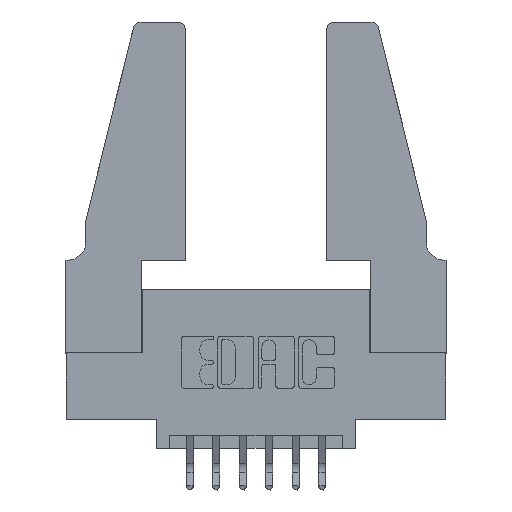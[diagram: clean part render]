
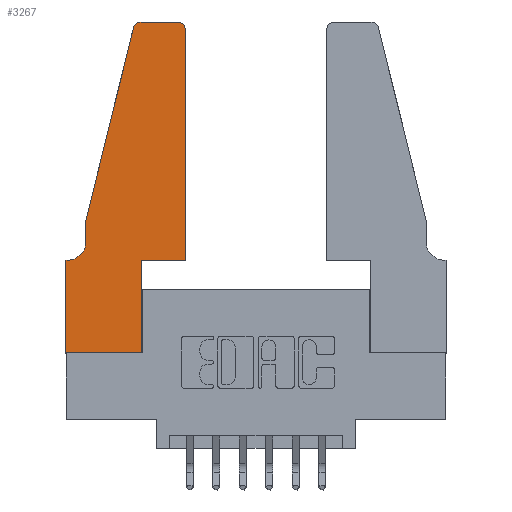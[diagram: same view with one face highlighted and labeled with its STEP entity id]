
A CAD part, top view. The second image highlights one B-rep face of the part: STEP entity #3267.
In plain terms, the highlighted planar face has unit normal (0, 0, 1).
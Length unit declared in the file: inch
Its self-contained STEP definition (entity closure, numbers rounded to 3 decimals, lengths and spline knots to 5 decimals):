
#171 = VECTOR ( 'NONE', #5055, 39.37008 ) ;
#303 = CARTESIAN_POINT ( 'NONE',  ( 0.4505, 1.22, 0.37 ) ) ;
#331 = CARTESIAN_POINT ( 'NONE',  ( 0.4505, 0.35, 0.37 ) ) ;
#343 = VERTEX_POINT ( 'NONE', #2088 ) ;
#432 = CARTESIAN_POINT ( 'NONE',  ( 0.284, 1.25, 0.37 ) ) ;
#476 = DIRECTION ( 'NONE',  ( 1., 0., 0. ) ) ;
#612 = CARTESIAN_POINT ( 'NONE',  ( 0.0055, 0.35, 0.37 ) ) ;
#624 = EDGE_CURVE ( 'NONE', #7523, #343, #2454, .T. ) ;
#1368 = EDGE_CURVE ( 'NONE', #3837, #6084, #7734, .T. ) ;
#1468 = DIRECTION ( 'NONE',  ( 0., 0., 1. ) ) ;
#1551 = VECTOR ( 'NONE', #6899, 39.37008 ) ;
#1742 = CIRCLE ( 'NONE', #3363, 0.03 ) ;
#1766 = LINE ( 'NONE', #4999, #3747 ) ;
#1780 = VERTEX_POINT ( 'NONE', #7003 ) ;
#1866 = ORIENTED_EDGE ( 'NONE', *, *, #7476, .T. ) ;
#2088 = CARTESIAN_POINT ( 'NONE',  ( 0.2865, 0.35, 0.37 ) ) ;
#2177 = DIRECTION ( 'NONE',  ( 0., 0., -1. ) ) ;
#2454 = LINE ( 'NONE', #7341, #4933 ) ;
#2511 = VECTOR ( 'NONE', #7193, 39.37008 ) ;
#2531 = ORIENTED_EDGE ( 'NONE', *, *, #624, .T. ) ;
#2634 = CARTESIAN_POINT ( 'NONE',  ( 0., 0., 0.37 ) ) ;
#2640 = LINE ( 'NONE', #2634, #2511 ) ;
#2693 = ORIENTED_EDGE ( 'NONE', *, *, #7391, .T. ) ;
#2748 = VERTEX_POINT ( 'NONE', #303 ) ;
#2749 = VERTEX_POINT ( 'NONE', #432 ) ;
#3013 = CARTESIAN_POINT ( 'NONE',  ( 0.25487, 1.22718, 0.37 ) ) ;
#3137 = DIRECTION ( 'NONE',  ( 1., 0., 0. ) ) ;
#3149 = DIRECTION ( 'NONE',  ( 0., 0., 1. ) ) ;
#3152 = DIRECTION ( 'NONE',  ( 0., 0., 1. ) ) ;
#3267 = ADVANCED_FACE ( 'NONE', ( #4009 ), #7244, .T. ) ;
#3281 = DIRECTION ( 'NONE',  ( 0., 1., 0. ) ) ;
#3363 = AXIS2_PLACEMENT_3D ( 'NONE', #7113, #1468, #7999 ) ;
#3400 = EDGE_LOOP ( 'NONE', ( #2693, #9396, #3849, #4908, #10937, #6862, #5491, #1866, #2531, #3650, #6677, #7152 ) ) ;
#3415 = EDGE_CURVE ( 'NONE', #7192, #3526, #6577, .T. ) ;
#3526 = VERTEX_POINT ( 'NONE', #7052 ) ;
#3606 = CARTESIAN_POINT ( 'NONE',  ( 0.2865, 0., 0.37 ) ) ;
#3614 = CARTESIAN_POINT ( 'NONE',  ( 0.0755, 0.35, 0.37 ) ) ;
#3650 = ORIENTED_EDGE ( 'NONE', *, *, #8264, .T. ) ;
#3747 = VECTOR ( 'NONE', #5887, 39.37008 ) ;
#3837 = VERTEX_POINT ( 'NONE', #8348 ) ;
#3849 = ORIENTED_EDGE ( 'NONE', *, *, #3415, .T. ) ;
#4009 = FACE_OUTER_BOUND ( 'NONE', #3400, .T. ) ;
#4021 = EDGE_CURVE ( 'NONE', #3526, #3837, #5422, .T. ) ;
#4097 = AXIS2_PLACEMENT_3D ( 'NONE', #7837, #2177, #8712 ) ;
#4147 = CARTESIAN_POINT ( 'NONE',  ( 0.0755, 0.5, 0.37 ) ) ;
#4204 = VERTEX_POINT ( 'NONE', #331 ) ;
#4529 = VERTEX_POINT ( 'NONE', #10191 ) ;
#4573 = AXIS2_PLACEMENT_3D ( 'NONE', #7260, #3152, #3137 ) ;
#4718 = CARTESIAN_POINT ( 'NONE',  ( 0.4505, 0.35, 0.37 ) ) ;
#4908 = ORIENTED_EDGE ( 'NONE', *, *, #4021, .T. ) ;
#4933 = VECTOR ( 'NONE', #3281, 39.37008 ) ;
#4999 = CARTESIAN_POINT ( 'NONE',  ( 0.4505, 0.35, 0.37 ) ) ;
#5055 = DIRECTION ( 'NONE',  ( 0., -1., 0. ) ) ;
#5067 = CARTESIAN_POINT ( 'NONE',  ( 0.0755, 0.5, 0.37 ) ) ;
#5356 = CIRCLE ( 'NONE', #7785, 0.03 ) ;
#5409 = EDGE_CURVE ( 'NONE', #1780, #6650, #2640, .T. ) ;
#5422 = LINE ( 'NONE', #4147, #171 ) ;
#5449 = VECTOR ( 'NONE', #6157, 39.37008 ) ;
#5491 = ORIENTED_EDGE ( 'NONE', *, *, #5409, .T. ) ;
#5887 = DIRECTION ( 'NONE',  ( 0., 1., 0. ) ) ;
#6084 = VERTEX_POINT ( 'NONE', #612 ) ;
#6157 = DIRECTION ( 'NONE',  ( -1., 0., 0. ) ) ;
#6577 = LINE ( 'NONE', #5067, #1551 ) ;
#6650 = VERTEX_POINT ( 'NONE', #10327 ) ;
#6654 = EDGE_CURVE ( 'NONE', #4204, #2748, #1766, .T. ) ;
#6677 = ORIENTED_EDGE ( 'NONE', *, *, #6654, .T. ) ;
#6862 = ORIENTED_EDGE ( 'NONE', *, *, #8697, .T. ) ;
#6899 = DIRECTION ( 'NONE',  ( -0.239, -0.971, 0. ) ) ;
#7003 = CARTESIAN_POINT ( 'NONE',  ( 0., 0.35, 0.37 ) ) ;
#7052 = CARTESIAN_POINT ( 'NONE',  ( 0.0755, 0.5, 0.37 ) ) ;
#7113 = CARTESIAN_POINT ( 'NONE',  ( 0.284, 1.22, 0.37 ) ) ;
#7152 = ORIENTED_EDGE ( 'NONE', *, *, #11967, .T. ) ;
#7192 = VERTEX_POINT ( 'NONE', #3013 ) ;
#7193 = DIRECTION ( 'NONE',  ( 0., -1., 0. ) ) ;
#7244 = PLANE ( 'NONE',  #4573 ) ;
#7260 = CARTESIAN_POINT ( 'NONE',  ( 0., 0.35, 0.37 ) ) ;
#7289 = LINE ( 'NONE', #11471, #5449 ) ;
#7341 = CARTESIAN_POINT ( 'NONE',  ( 0.2865, 0.35, 0.37 ) ) ;
#7391 = EDGE_CURVE ( 'NONE', #4529, #2749, #7289, .T. ) ;
#7408 = DIRECTION ( 'NONE',  ( 1., 0., 0. ) ) ;
#7428 = EDGE_CURVE ( 'NONE', #2749, #7192, #1742, .T. ) ;
#7476 = EDGE_CURVE ( 'NONE', #6650, #7523, #10875, .T. ) ;
#7523 = VERTEX_POINT ( 'NONE', #3606 ) ;
#7734 = CIRCLE ( 'NONE', #4097, 0.07 ) ;
#7785 = AXIS2_PLACEMENT_3D ( 'NONE', #8545, #3149, #9441 ) ;
#7837 = CARTESIAN_POINT ( 'NONE',  ( 0.0055, 0.42, 0.37 ) ) ;
#7999 = DIRECTION ( 'NONE',  ( 1., 0., 0. ) ) ;
#8264 = EDGE_CURVE ( 'NONE', #343, #4204, #9498, .T. ) ;
#8348 = CARTESIAN_POINT ( 'NONE',  ( 0.0755, 0.42, 0.37 ) ) ;
#8545 = CARTESIAN_POINT ( 'NONE',  ( 0.4205, 1.22, 0.37 ) ) ;
#8697 = EDGE_CURVE ( 'NONE', #6084, #1780, #9488, .T. ) ;
#8712 = DIRECTION ( 'NONE',  ( -1., 0., 0. ) ) ;
#9396 = ORIENTED_EDGE ( 'NONE', *, *, #7428, .T. ) ;
#9441 = DIRECTION ( 'NONE',  ( 1., 0., 0. ) ) ;
#9488 = LINE ( 'NONE', #3614, #10032 ) ;
#9498 = LINE ( 'NONE', #4718, #11852 ) ;
#9903 = DIRECTION ( 'NONE',  ( -1., 0., 0. ) ) ;
#10032 = VECTOR ( 'NONE', #9903, 39.37008 ) ;
#10191 = CARTESIAN_POINT ( 'NONE',  ( 0.4205, 1.25, 0.37 ) ) ;
#10327 = CARTESIAN_POINT ( 'NONE',  ( 0., 0., 0.37 ) ) ;
#10587 = VECTOR ( 'NONE', #476, 39.37008 ) ;
#10875 = LINE ( 'NONE', #11601, #10587 ) ;
#10937 = ORIENTED_EDGE ( 'NONE', *, *, #1368, .T. ) ;
#11471 = CARTESIAN_POINT ( 'NONE',  ( 0.2605, 1.25, 0.37 ) ) ;
#11601 = CARTESIAN_POINT ( 'NONE',  ( 0., 0., 0.37 ) ) ;
#11852 = VECTOR ( 'NONE', #7408, 39.37008 ) ;
#11967 = EDGE_CURVE ( 'NONE', #2748, #4529, #5356, .T. ) ;
